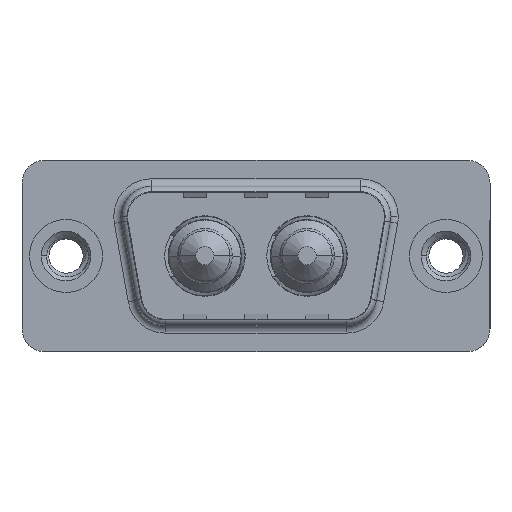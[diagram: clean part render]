
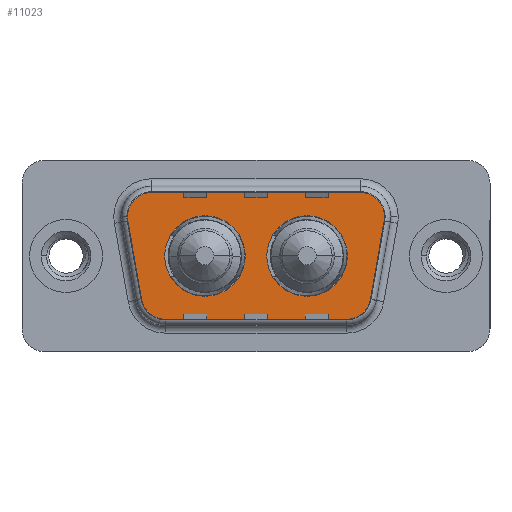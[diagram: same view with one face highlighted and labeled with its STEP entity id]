
A CAD part, top view. The second image highlights one B-rep face of the part: STEP entity #11023.
In plain terms, the highlighted planar face has unit normal (0, 0, 1).
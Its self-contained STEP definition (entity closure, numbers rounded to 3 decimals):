
#36 = CARTESIAN_POINT ( 'NONE',  ( 3.466, 2.553, 0. ) ) ;
#469 = AXIS2_PLACEMENT_3D ( 'NONE', #555, #8503, #3269 ) ;
#555 = CARTESIAN_POINT ( 'NONE',  ( 18.541, -2.9, 0. ) ) ;
#570 = CIRCLE ( 'NONE', #9247, 2.65 ) ;
#650 = VERTEX_POINT ( 'NONE', #3073 ) ;
#661 = CARTESIAN_POINT ( 'NONE',  ( 6.459, -4.9, 0. ) ) ;
#836 = EDGE_CURVE ( 'NONE', #4151, #8927, #570, .T. ) ;
#1037 = DIRECTION ( 'NONE',  ( -1., 0., 0. ) ) ;
#1463 = DIRECTION ( 'NONE',  ( 0., 0., 1. ) ) ;
#1478 = VERTEX_POINT ( 'NONE', #3068 ) ;
#1494 = LINE ( 'NONE', #10546, #3892 ) ;
#1503 = CARTESIAN_POINT ( 'NONE',  ( 9.14, 0., 0. ) ) ;
#1540 = EDGE_CURVE ( 'NONE', #4087, #8480, #6286, .T. ) ;
#1541 = EDGE_CURVE ( 'NONE', #3605, #6084, #1551, .T. ) ;
#1551 = CIRCLE ( 'NONE', #5845, 2. ) ;
#1585 = ORIENTED_EDGE ( 'NONE', *, *, #9021, .F. ) ;
#1765 = EDGE_CURVE ( 'NONE', #1478, #3605, #7210, .T. ) ;
#1786 = CARTESIAN_POINT ( 'NONE',  ( 4.489, -3.247, 0. ) ) ;
#1940 = CARTESIAN_POINT ( 'NONE',  ( 18.51, 0., 0. ) ) ;
#2090 = CARTESIAN_POINT ( 'NONE',  ( 15.86, 0., 0. ) ) ;
#2125 = ORIENTED_EDGE ( 'NONE', *, *, #4474, .T. ) ;
#2239 = VECTOR ( 'NONE', #10458, 1000. ) ;
#2328 = DIRECTION ( 'NONE',  ( 0., 0., 1. ) ) ;
#2341 = EDGE_CURVE ( 'NONE', #8818, #650, #6145, .T. ) ;
#2428 = DIRECTION ( 'NONE',  ( 0., 0., 1. ) ) ;
#2807 = EDGE_LOOP ( 'NONE', ( #7242, #10767, #3339, #10562, #7499, #11394, #2125, #5842, #8618 ) ) ;
#2927 = FACE_BOUND ( 'NONE', #3498, .T. ) ;
#2984 = DIRECTION ( 'NONE',  ( 1., 0., 0. ) ) ;
#3068 = CARTESIAN_POINT ( 'NONE',  ( 20.511, -3.247, 0. ) ) ;
#3073 = CARTESIAN_POINT ( 'NONE',  ( 6.459, -4.9, 0. ) ) ;
#3148 = CIRCLE ( 'NONE', #3602, 2. ) ;
#3269 = DIRECTION ( 'NONE',  ( 1., 0., 0. ) ) ;
#3339 = ORIENTED_EDGE ( 'NONE', *, *, #1541, .T. ) ;
#3498 = EDGE_LOOP ( 'NONE', ( #1585, #11347 ) ) ;
#3499 = AXIS2_PLACEMENT_3D ( 'NONE', #10763, #5012, #6364 ) ;
#3536 = DIRECTION ( 'NONE',  ( -1., 0., 0. ) ) ;
#3570 = VECTOR ( 'NONE', #6866, 1000. ) ;
#3602 = AXIS2_PLACEMENT_3D ( 'NONE', #7689, #2428, #8570 ) ;
#3605 = VERTEX_POINT ( 'NONE', #5160 ) ;
#3719 = CIRCLE ( 'NONE', #4436, 2. ) ;
#3892 = VECTOR ( 'NONE', #10431, 1000. ) ;
#3981 = CIRCLE ( 'NONE', #4516, 2.65 ) ;
#4066 = AXIS2_PLACEMENT_3D ( 'NONE', #7192, #7043, #6846 ) ;
#4087 = VERTEX_POINT ( 'NONE', #6559 ) ;
#4147 = PLANE ( 'NONE',  #469 ) ;
#4149 = DIRECTION ( 'NONE',  ( 1., 0., 0. ) ) ;
#4151 = VERTEX_POINT ( 'NONE', #10104 ) ;
#4161 = AXIS2_PLACEMENT_3D ( 'NONE', #10061, #6845, #1037 ) ;
#4166 = CIRCLE ( 'NONE', #3499, 2. ) ;
#4378 = EDGE_CURVE ( 'NONE', #8480, #4087, #4739, .T. ) ;
#4436 = AXIS2_PLACEMENT_3D ( 'NONE', #5118, #11241, #5989 ) ;
#4474 = EDGE_CURVE ( 'NONE', #11318, #8818, #1494, .T. ) ;
#4516 = AXIS2_PLACEMENT_3D ( 'NONE', #2090, #8232, #2984 ) ;
#4700 = LINE ( 'NONE', #11481, #9015 ) ;
#4704 = VERTEX_POINT ( 'NONE', #8722 ) ;
#4739 = CIRCLE ( 'NONE', #5593, 2.65 ) ;
#5001 = EDGE_CURVE ( 'NONE', #6084, #4704, #4166, .T. ) ;
#5012 = DIRECTION ( 'NONE',  ( 0., 0., 1. ) ) ;
#5018 = EDGE_LOOP ( 'NONE', ( #9284, #9835 ) ) ;
#5067 = DIRECTION ( 'NONE',  ( 1., 0., 0. ) ) ;
#5118 = CARTESIAN_POINT ( 'NONE',  ( 5.436, 2.9, 0. ) ) ;
#5160 = CARTESIAN_POINT ( 'NONE',  ( 21.534, 2.553, 0. ) ) ;
#5286 = CARTESIAN_POINT ( 'NONE',  ( 21.564, 2.9, 0. ) ) ;
#5355 = FACE_BOUND ( 'NONE', #5018, .T. ) ;
#5593 = AXIS2_PLACEMENT_3D ( 'NONE', #1503, #1463, #5067 ) ;
#5842 = ORIENTED_EDGE ( 'NONE', *, *, #2341, .T. ) ;
#5845 = AXIS2_PLACEMENT_3D ( 'NONE', #8406, #2328, #6141 ) ;
#5937 = EDGE_CURVE ( 'NONE', #7393, #1478, #3148, .T. ) ;
#5989 = DIRECTION ( 'NONE',  ( 1., 0., 0. ) ) ;
#6084 = VERTEX_POINT ( 'NONE', #5286 ) ;
#6141 = DIRECTION ( 'NONE',  ( -1., 0., 0. ) ) ;
#6145 = CIRCLE ( 'NONE', #4161, 2. ) ;
#6286 = CIRCLE ( 'NONE', #4066, 2.65 ) ;
#6364 = DIRECTION ( 'NONE',  ( -1., 0., 0. ) ) ;
#6559 = CARTESIAN_POINT ( 'NONE',  ( 11.79, 0., 0. ) ) ;
#6845 = DIRECTION ( 'NONE',  ( 0., 0., 1. ) ) ;
#6846 = DIRECTION ( 'NONE',  ( 1., 0., 0. ) ) ;
#6866 = DIRECTION ( 'NONE',  ( 1., 0., 0. ) ) ;
#7043 = DIRECTION ( 'NONE',  ( 0., 0., 1. ) ) ;
#7071 = CARTESIAN_POINT ( 'NONE',  ( 21.534, 2.553, 0. ) ) ;
#7192 = CARTESIAN_POINT ( 'NONE',  ( 9.14, 0., 0. ) ) ;
#7210 = LINE ( 'NONE', #7071, #2239 ) ;
#7242 = ORIENTED_EDGE ( 'NONE', *, *, #5937, .T. ) ;
#7393 = VERTEX_POINT ( 'NONE', #10505 ) ;
#7443 = CARTESIAN_POINT ( 'NONE',  ( 15.86, 0., 0. ) ) ;
#7499 = ORIENTED_EDGE ( 'NONE', *, *, #8084, .T. ) ;
#7689 = CARTESIAN_POINT ( 'NONE',  ( 18.541, -2.9, 0. ) ) ;
#7931 = EDGE_CURVE ( 'NONE', #9166, #11318, #3719, .T. ) ;
#8084 = EDGE_CURVE ( 'NONE', #4704, #9166, #4700, .T. ) ;
#8221 = EDGE_CURVE ( 'NONE', #650, #7393, #10289, .T. ) ;
#8232 = DIRECTION ( 'NONE',  ( 0., 0., 1. ) ) ;
#8244 = DIRECTION ( 'NONE',  ( 0., 0., 1. ) ) ;
#8406 = CARTESIAN_POINT ( 'NONE',  ( 19.564, 2.9, 0. ) ) ;
#8480 = VERTEX_POINT ( 'NONE', #9805 ) ;
#8503 = DIRECTION ( 'NONE',  ( 0., 0., 1. ) ) ;
#8570 = DIRECTION ( 'NONE',  ( 1., 0., 0. ) ) ;
#8618 = ORIENTED_EDGE ( 'NONE', *, *, #8221, .T. ) ;
#8640 = CARTESIAN_POINT ( 'NONE',  ( 5.436, 4.9, 0. ) ) ;
#8722 = CARTESIAN_POINT ( 'NONE',  ( 19.564, 4.9, 0. ) ) ;
#8818 = VERTEX_POINT ( 'NONE', #1786 ) ;
#8927 = VERTEX_POINT ( 'NONE', #1940 ) ;
#9015 = VECTOR ( 'NONE', #3536, 1000. ) ;
#9021 = EDGE_CURVE ( 'NONE', #8927, #4151, #3981, .T. ) ;
#9166 = VERTEX_POINT ( 'NONE', #8640 ) ;
#9247 = AXIS2_PLACEMENT_3D ( 'NONE', #7443, #8244, #4149 ) ;
#9284 = ORIENTED_EDGE ( 'NONE', *, *, #1540, .F. ) ;
#9805 = CARTESIAN_POINT ( 'NONE',  ( 6.49, 0., 0. ) ) ;
#9835 = ORIENTED_EDGE ( 'NONE', *, *, #4378, .F. ) ;
#9955 = FACE_OUTER_BOUND ( 'NONE', #2807, .T. ) ;
#10061 = CARTESIAN_POINT ( 'NONE',  ( 6.459, -2.9, 0. ) ) ;
#10104 = CARTESIAN_POINT ( 'NONE',  ( 13.21, 0., 0. ) ) ;
#10289 = LINE ( 'NONE', #661, #3570 ) ;
#10431 = DIRECTION ( 'NONE',  ( 0.174, -0.985, 0. ) ) ;
#10458 = DIRECTION ( 'NONE',  ( 0.174, 0.985, 0. ) ) ;
#10505 = CARTESIAN_POINT ( 'NONE',  ( 18.541, -4.9, 0. ) ) ;
#10546 = CARTESIAN_POINT ( 'NONE',  ( 3.466, 2.553, 0. ) ) ;
#10562 = ORIENTED_EDGE ( 'NONE', *, *, #5001, .T. ) ;
#10763 = CARTESIAN_POINT ( 'NONE',  ( 19.564, 2.9, 0. ) ) ;
#10767 = ORIENTED_EDGE ( 'NONE', *, *, #1765, .T. ) ;
#11023 = ADVANCED_FACE ( 'NONE', ( #2927, #5355, #9955 ), #4147, .T. ) ;
#11241 = DIRECTION ( 'NONE',  ( 0., 0., 1. ) ) ;
#11318 = VERTEX_POINT ( 'NONE', #36 ) ;
#11347 = ORIENTED_EDGE ( 'NONE', *, *, #836, .F. ) ;
#11394 = ORIENTED_EDGE ( 'NONE', *, *, #7931, .T. ) ;
#11481 = CARTESIAN_POINT ( 'NONE',  ( 5.436, 4.9, 0. ) ) ;
